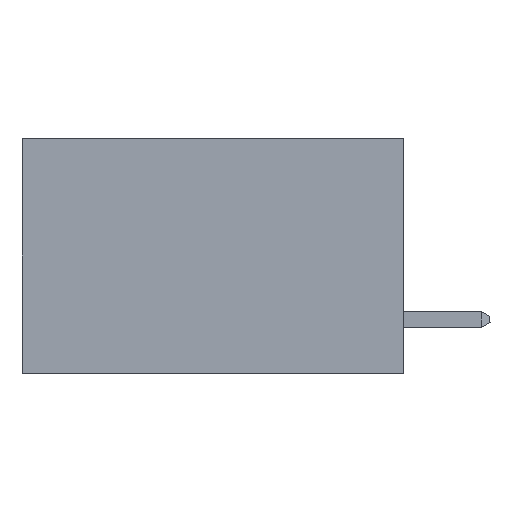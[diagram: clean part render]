
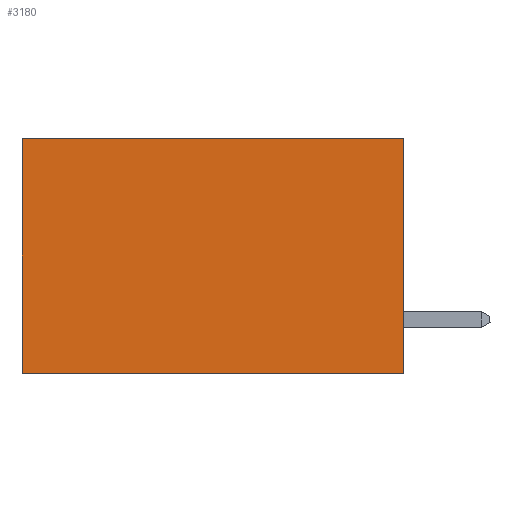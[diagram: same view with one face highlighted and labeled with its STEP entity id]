
A CAD part, left-side view. The second image highlights one B-rep face of the part: STEP entity #3180.
In plain terms, the highlighted planar face has unit normal (-1, 0, 0).
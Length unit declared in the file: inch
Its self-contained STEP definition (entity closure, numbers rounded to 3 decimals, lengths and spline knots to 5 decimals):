
#824 = VERTEX_POINT ( 'NONE', #7225 ) ;
#3180 = ADVANCED_FACE ( 'NONE', ( #31360 ), #20509, .F. ) ;
#5383 = EDGE_CURVE ( 'NONE', #824, #15021, #32640, .T. ) ;
#6303 = CARTESIAN_POINT ( 'NONE',  ( 0.2875, 0., -0.37 ) ) ;
#6412 = CARTESIAN_POINT ( 'NONE',  ( 0.2875, 0., -0.37 ) ) ;
#6992 = AXIS2_PLACEMENT_3D ( 'NONE', #20930, #25548, #28234 ) ;
#7225 = CARTESIAN_POINT ( 'NONE',  ( 0.2875, 0., 0. ) ) ;
#9469 = DIRECTION ( 'NONE',  ( 0., 1., 0. ) ) ;
#11272 = VERTEX_POINT ( 'NONE', #6412 ) ;
#11666 = CARTESIAN_POINT ( 'NONE',  ( 0.2875, 0.6, 0. ) ) ;
#12019 = VECTOR ( 'NONE', #9469, 39.37008 ) ;
#14078 = CARTESIAN_POINT ( 'NONE',  ( 0.2875, 0., 0. ) ) ;
#14351 = DIRECTION ( 'NONE',  ( 0., 0., -1. ) ) ;
#14660 = EDGE_CURVE ( 'NONE', #15021, #36710, #31508, .T. ) ;
#15021 = VERTEX_POINT ( 'NONE', #11666 ) ;
#16695 = ORIENTED_EDGE ( 'NONE', *, *, #5383, .T. ) ;
#19158 = EDGE_CURVE ( 'NONE', #824, #11272, #40437, .T. ) ;
#19842 = EDGE_LOOP ( 'NONE', ( #37894, #33688, #38506, #16695 ) ) ;
#20458 = CARTESIAN_POINT ( 'NONE',  ( 0.2875, 0.6, 0. ) ) ;
#20509 = PLANE ( 'NONE',  #6992 ) ;
#20930 = CARTESIAN_POINT ( 'NONE',  ( 0.2875, 0., 0. ) ) ;
#21048 = DIRECTION ( 'NONE',  ( 0., 0., -1. ) ) ;
#21946 = VECTOR ( 'NONE', #27490, 39.37008 ) ;
#25548 = DIRECTION ( 'NONE',  ( 1., 0., 0. ) ) ;
#27337 = LINE ( 'NONE', #6303, #12019 ) ;
#27490 = DIRECTION ( 'NONE',  ( 0., 1., 0. ) ) ;
#28234 = DIRECTION ( 'NONE',  ( 0., 0., -1. ) ) ;
#28729 = VECTOR ( 'NONE', #21048, 39.37008 ) ;
#30430 = CARTESIAN_POINT ( 'NONE',  ( 0.2875, 0.6, -0.37 ) ) ;
#31360 = FACE_OUTER_BOUND ( 'NONE', #19842, .T. ) ;
#31508 = LINE ( 'NONE', #20458, #34904 ) ;
#32640 = LINE ( 'NONE', #35926, #21946 ) ;
#33688 = ORIENTED_EDGE ( 'NONE', *, *, #37535, .F. ) ;
#34904 = VECTOR ( 'NONE', #14351, 39.37008 ) ;
#35926 = CARTESIAN_POINT ( 'NONE',  ( 0.2875, 0., 0. ) ) ;
#36710 = VERTEX_POINT ( 'NONE', #30430 ) ;
#37535 = EDGE_CURVE ( 'NONE', #11272, #36710, #27337, .T. ) ;
#37894 = ORIENTED_EDGE ( 'NONE', *, *, #14660, .T. ) ;
#38506 = ORIENTED_EDGE ( 'NONE', *, *, #19158, .F. ) ;
#40437 = LINE ( 'NONE', #14078, #28729 ) ;
